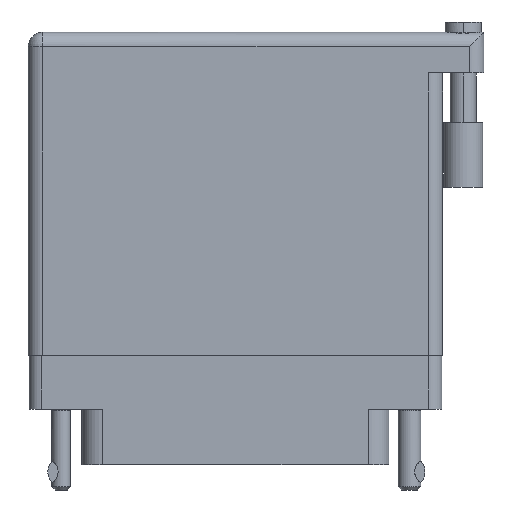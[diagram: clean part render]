
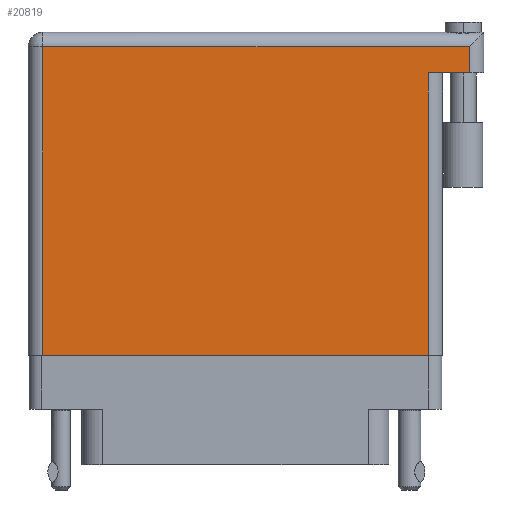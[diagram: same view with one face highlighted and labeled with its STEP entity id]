
A CAD part, front view. The second image highlights one B-rep face of the part: STEP entity #20819.
In plain terms, the highlighted face is planar.
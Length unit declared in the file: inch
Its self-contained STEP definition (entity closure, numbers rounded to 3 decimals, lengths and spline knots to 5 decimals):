
#1008 = VERTEX_POINT ( 'NONE', #16810 ) ;
#1883 = VERTEX_POINT ( 'NONE', #22159 ) ;
#2023 = DIRECTION ( 'NONE',  ( 0., 1., 0. ) ) ;
#2226 = CARTESIAN_POINT ( 'NONE',  ( 0., 1.496, 0. ) ) ;
#2843 = EDGE_CURVE ( 'NONE', #5643, #26142, #11095, .T. ) ;
#3851 = DIRECTION ( 'NONE',  ( 0., 1., 0. ) ) ;
#4204 = CARTESIAN_POINT ( 'NONE',  ( 0.07, 0., 0. ) ) ;
#5328 = CARTESIAN_POINT ( 'NONE',  ( 2.138, 1.496, 0. ) ) ;
#5643 = VERTEX_POINT ( 'NONE', #12312 ) ;
#7378 = CARTESIAN_POINT ( 'NONE',  ( 2.138, 1.566, 0. ) ) ;
#7870 = LINE ( 'NONE', #7378, #37968 ) ;
#8399 = VECTOR ( 'NONE', #10605, 39.37008 ) ;
#9607 = DIRECTION ( 'NONE',  ( -1., 0., 0. ) ) ;
#10563 = CARTESIAN_POINT ( 'NONE',  ( 2.138, 1.369, 0. ) ) ;
#10605 = DIRECTION ( 'NONE',  ( 1., 0., 0. ) ) ;
#10703 = EDGE_CURVE ( 'NONE', #1008, #1883, #37046, .T. ) ;
#11095 = LINE ( 'NONE', #4204, #23245 ) ;
#11850 = DIRECTION ( 'NONE',  ( -1., 0., 0. ) ) ;
#12312 = CARTESIAN_POINT ( 'NONE',  ( 0.07, 1.496, 0. ) ) ;
#15132 = EDGE_CURVE ( 'NONE', #17525, #1883, #33603, .T. ) ;
#16810 = CARTESIAN_POINT ( 'NONE',  ( 1.938, 0., 0. ) ) ;
#17525 = VERTEX_POINT ( 'NONE', #10563 ) ;
#18205 = CARTESIAN_POINT ( 'NONE',  ( 0., 0., 0. ) ) ;
#18907 = EDGE_CURVE ( 'NONE', #26142, #1008, #24608, .T. ) ;
#19285 = CARTESIAN_POINT ( 'NONE',  ( 2.208, 1.369, 0. ) ) ;
#19392 = EDGE_CURVE ( 'NONE', #39065, #5643, #34428, .T. ) ;
#20819 = ADVANCED_FACE ( 'NONE', ( #47710 ), #23253, .F. ) ;
#21011 = ORIENTED_EDGE ( 'NONE', *, *, #15132, .F. ) ;
#22023 = EDGE_LOOP ( 'NONE', ( #38238, #37904, #21011, #23741, #40505, #37111 ) ) ;
#22159 = CARTESIAN_POINT ( 'NONE',  ( 1.938, 1.369, 0. ) ) ;
#22422 = CARTESIAN_POINT ( 'NONE',  ( 0.07, 0., 0. ) ) ;
#23245 = VECTOR ( 'NONE', #29540, 39.37008 ) ;
#23253 = PLANE ( 'NONE',  #24602 ) ;
#23741 = ORIENTED_EDGE ( 'NONE', *, *, #26706, .T. ) ;
#24602 = AXIS2_PLACEMENT_3D ( 'NONE', #34410, #26350, #41672 ) ;
#24608 = LINE ( 'NONE', #18205, #8399 ) ;
#26142 = VERTEX_POINT ( 'NONE', #22422 ) ;
#26350 = DIRECTION ( 'NONE',  ( 0., 0., -1. ) ) ;
#26706 = EDGE_CURVE ( 'NONE', #17525, #39065, #7870, .T. ) ;
#27840 = CARTESIAN_POINT ( 'NONE',  ( 1.938, 1.369, 0. ) ) ;
#29540 = DIRECTION ( 'NONE',  ( 0., -1., 0. ) ) ;
#31847 = VECTOR ( 'NONE', #11850, 39.37008 ) ;
#33603 = LINE ( 'NONE', #19285, #31847 ) ;
#34410 = CARTESIAN_POINT ( 'NONE',  ( 0., 1.566, 0. ) ) ;
#34428 = LINE ( 'NONE', #2226, #40199 ) ;
#37046 = LINE ( 'NONE', #27840, #43391 ) ;
#37111 = ORIENTED_EDGE ( 'NONE', *, *, #2843, .T. ) ;
#37904 = ORIENTED_EDGE ( 'NONE', *, *, #10703, .T. ) ;
#37968 = VECTOR ( 'NONE', #3851, 39.37008 ) ;
#38238 = ORIENTED_EDGE ( 'NONE', *, *, #18907, .T. ) ;
#39065 = VERTEX_POINT ( 'NONE', #5328 ) ;
#40199 = VECTOR ( 'NONE', #9607, 39.37008 ) ;
#40505 = ORIENTED_EDGE ( 'NONE', *, *, #19392, .T. ) ;
#41672 = DIRECTION ( 'NONE',  ( -1., 0., 0. ) ) ;
#43391 = VECTOR ( 'NONE', #2023, 39.37008 ) ;
#47710 = FACE_OUTER_BOUND ( 'NONE', #22023, .T. ) ;
